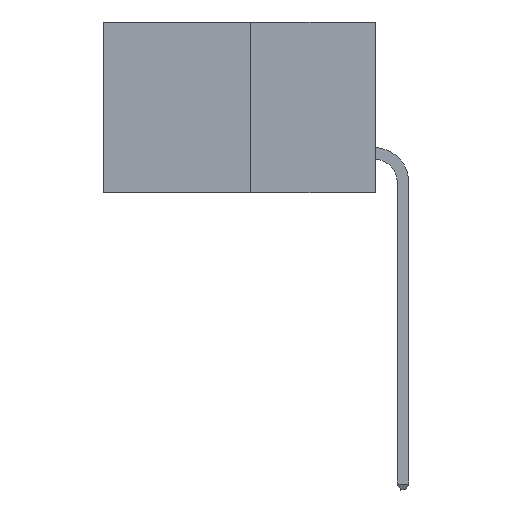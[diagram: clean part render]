
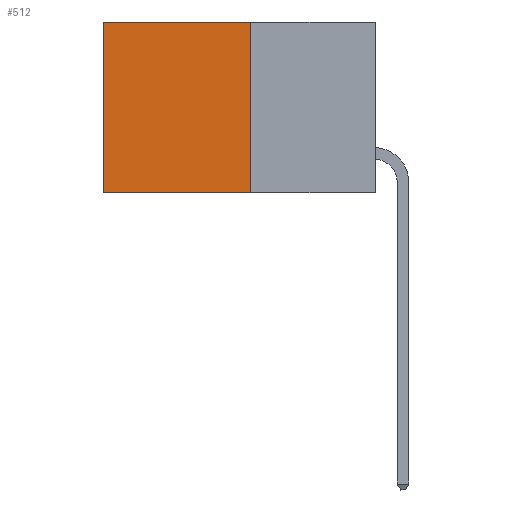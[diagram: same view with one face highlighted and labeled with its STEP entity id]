
A CAD part, left-side view. The second image highlights one B-rep face of the part: STEP entity #512.
In plain terms, the highlighted planar face has unit normal (-1, 0, 0).
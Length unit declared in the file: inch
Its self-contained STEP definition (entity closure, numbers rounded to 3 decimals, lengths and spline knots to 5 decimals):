
#196 = AXIS2_PLACEMENT_3D ( 'NONE', #7287, #7869, #5817 ) ;
#226 = CARTESIAN_POINT ( 'NONE',  ( 0.277, 0.27, 0. ) ) ;
#437 = ORIENTED_EDGE ( 'NONE', *, *, #8934, .T. ) ;
#462 = PLANE ( 'NONE',  #196 ) ;
#507 = ORIENTED_EDGE ( 'NONE', *, *, #1821, .F. ) ;
#509 = ORIENTED_EDGE ( 'NONE', *, *, #9307, .F. ) ;
#512 = ADVANCED_FACE ( 'NONE', ( #894 ), #462, .F. ) ;
#521 = ORIENTED_EDGE ( 'NONE', *, *, #9657, .T. ) ;
#588 = VERTEX_POINT ( 'NONE', #2690 ) ;
#593 = DIRECTION ( 'NONE',  ( 0., 0., -1. ) ) ;
#894 = FACE_OUTER_BOUND ( 'NONE', #6248, .T. ) ;
#1821 = EDGE_CURVE ( 'NONE', #4568, #588, #7115, .T. ) ;
#2135 = LINE ( 'NONE', #10367, #6336 ) ;
#2465 = DIRECTION ( 'NONE',  ( 0., 1., 0. ) ) ;
#2674 = VECTOR ( 'NONE', #5501, 39.37008 ) ;
#2690 = CARTESIAN_POINT ( 'NONE',  ( 0.277, 0.59, -0.37 ) ) ;
#3136 = CARTESIAN_POINT ( 'NONE',  ( 0.277, 0.27, -0.37 ) ) ;
#3893 = LINE ( 'NONE', #10072, #5804 ) ;
#4457 = VERTEX_POINT ( 'NONE', #226 ) ;
#4568 = VERTEX_POINT ( 'NONE', #3136 ) ;
#4622 = CARTESIAN_POINT ( 'NONE',  ( 0.277, 0.27, -0.37 ) ) ;
#5501 = DIRECTION ( 'NONE',  ( 0., 1., 0. ) ) ;
#5562 = VECTOR ( 'NONE', #593, 39.37008 ) ;
#5734 = CARTESIAN_POINT ( 'NONE',  ( 0.277, 0.59, -0.37 ) ) ;
#5804 = VECTOR ( 'NONE', #6262, 39.37008 ) ;
#5817 = DIRECTION ( 'NONE',  ( 0., 0., -1. ) ) ;
#6248 = EDGE_LOOP ( 'NONE', ( #437, #507, #509, #521 ) ) ;
#6262 = DIRECTION ( 'NONE',  ( 0., 0., -1. ) ) ;
#6336 = VECTOR ( 'NONE', #2465, 39.37008 ) ;
#7115 = LINE ( 'NONE', #4622, #2674 ) ;
#7287 = CARTESIAN_POINT ( 'NONE',  ( 0.277, 0.27, -0.37 ) ) ;
#7514 = LINE ( 'NONE', #5734, #5562 ) ;
#7758 = CARTESIAN_POINT ( 'NONE',  ( 0.277, 0.59, 0. ) ) ;
#7869 = DIRECTION ( 'NONE',  ( 1., 0., 0. ) ) ;
#8934 = EDGE_CURVE ( 'NONE', #9212, #588, #7514, .T. ) ;
#9212 = VERTEX_POINT ( 'NONE', #7758 ) ;
#9307 = EDGE_CURVE ( 'NONE', #4457, #4568, #3893, .T. ) ;
#9657 = EDGE_CURVE ( 'NONE', #4457, #9212, #2135, .T. ) ;
#10072 = CARTESIAN_POINT ( 'NONE',  ( 0.277, 0.27, -0.37 ) ) ;
#10367 = CARTESIAN_POINT ( 'NONE',  ( 0.277, 0.27, 0. ) ) ;
